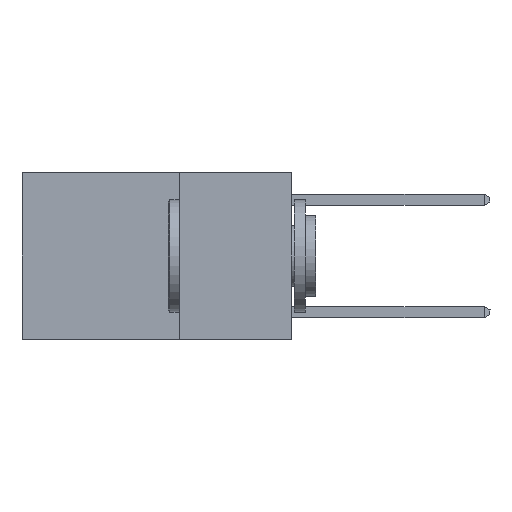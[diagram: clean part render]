
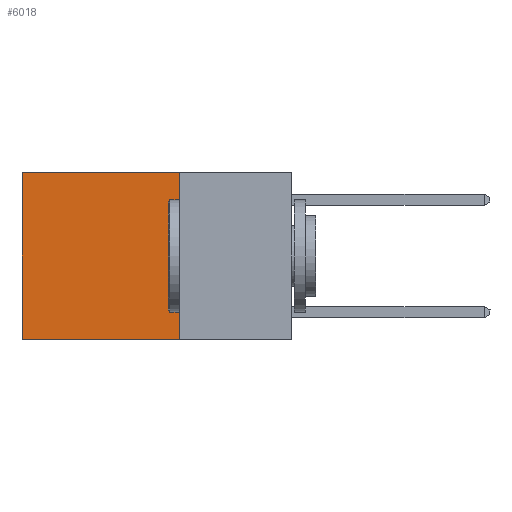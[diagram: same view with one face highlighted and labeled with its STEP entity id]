
A CAD part, left-side view. The second image highlights one B-rep face of the part: STEP entity #6018.
In plain terms, the highlighted planar face has unit normal (-1, 0, 0).
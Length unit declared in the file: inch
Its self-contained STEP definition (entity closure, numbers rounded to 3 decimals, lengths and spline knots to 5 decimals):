
#97 = DIRECTION ( 'NONE',  ( 0., 0., -1. ) ) ;
#129 = VECTOR ( 'NONE', #97, 39.37008 ) ;
#1518 = EDGE_CURVE ( 'NONE', #10697, #14276, #13831, .T. ) ;
#1801 = EDGE_CURVE ( 'NONE', #4300, #14276, #16587, .T. ) ;
#1914 = CARTESIAN_POINT ( 'NONE',  ( 0.2625, 0.25, 0. ) ) ;
#2072 = PLANE ( 'NONE',  #2802 ) ;
#2576 = EDGE_CURVE ( 'NONE', #13561, #4300, #5033, .T. ) ;
#2802 = AXIS2_PLACEMENT_3D ( 'NONE', #5256, #8469, #18964 ) ;
#3294 = CARTESIAN_POINT ( 'NONE',  ( 0.2625, 0.25, 0. ) ) ;
#3988 = EDGE_CURVE ( 'NONE', #13561, #10697, #10118, .T. ) ;
#4300 = VERTEX_POINT ( 'NONE', #13857 ) ;
#5033 = LINE ( 'NONE', #3294, #16817 ) ;
#5256 = CARTESIAN_POINT ( 'NONE',  ( 0.2625, 0.25, 0. ) ) ;
#5544 = VECTOR ( 'NONE', #9993, 39.37008 ) ;
#5981 = VECTOR ( 'NONE', #14857, 39.37008 ) ;
#6018 = ADVANCED_FACE ( 'NONE', ( #16150 ), #2072, .F. ) ;
#6678 = CARTESIAN_POINT ( 'NONE',  ( 0.2625, 0.6, -0.37 ) ) ;
#8469 = DIRECTION ( 'NONE',  ( 1., 0., 0. ) ) ;
#9013 = ORIENTED_EDGE ( 'NONE', *, *, #3988, .F. ) ;
#9405 = ORIENTED_EDGE ( 'NONE', *, *, #2576, .T. ) ;
#9578 = EDGE_LOOP ( 'NONE', ( #11730, #19701, #9013, #9405 ) ) ;
#9993 = DIRECTION ( 'NONE',  ( 0., 1., 0. ) ) ;
#10118 = LINE ( 'NONE', #19183, #5981 ) ;
#10697 = VERTEX_POINT ( 'NONE', #18577 ) ;
#11528 = CARTESIAN_POINT ( 'NONE',  ( 0.2625, 0.25, -0.37 ) ) ;
#11730 = ORIENTED_EDGE ( 'NONE', *, *, #1801, .T. ) ;
#13561 = VERTEX_POINT ( 'NONE', #1914 ) ;
#13831 = LINE ( 'NONE', #11528, #5544 ) ;
#13857 = CARTESIAN_POINT ( 'NONE',  ( 0.2625, 0.6, 0. ) ) ;
#14099 = CARTESIAN_POINT ( 'NONE',  ( 0.2625, 0.6, 0. ) ) ;
#14268 = DIRECTION ( 'NONE',  ( 0., 1., 0. ) ) ;
#14276 = VERTEX_POINT ( 'NONE', #6678 ) ;
#14857 = DIRECTION ( 'NONE',  ( 0., 0., -1. ) ) ;
#16150 = FACE_OUTER_BOUND ( 'NONE', #9578, .T. ) ;
#16587 = LINE ( 'NONE', #14099, #129 ) ;
#16817 = VECTOR ( 'NONE', #14268, 39.37008 ) ;
#18577 = CARTESIAN_POINT ( 'NONE',  ( 0.2625, 0.25, -0.37 ) ) ;
#18964 = DIRECTION ( 'NONE',  ( 0., 0., -1. ) ) ;
#19183 = CARTESIAN_POINT ( 'NONE',  ( 0.2625, 0.25, 0. ) ) ;
#19701 = ORIENTED_EDGE ( 'NONE', *, *, #1518, .F. ) ;
